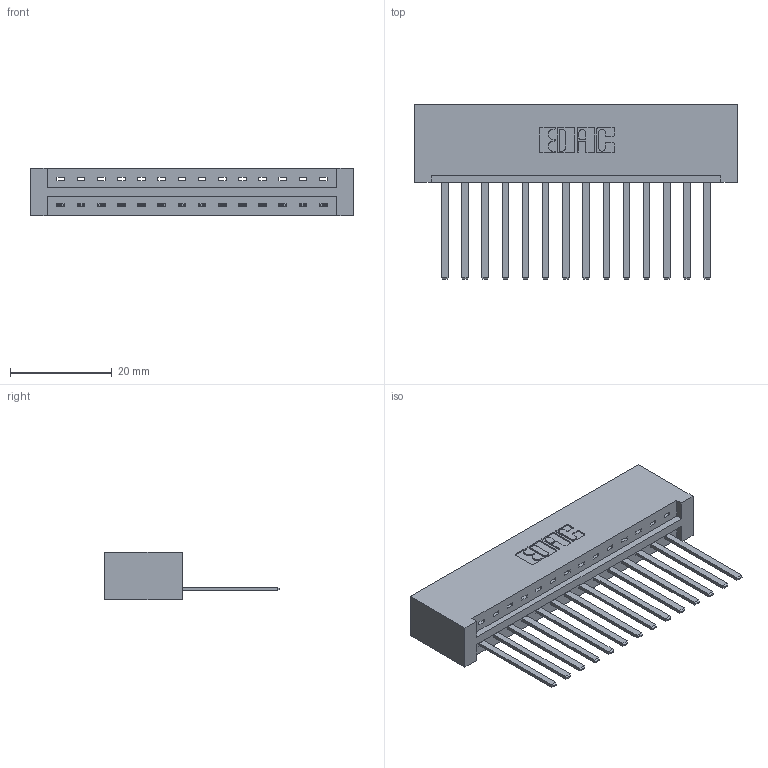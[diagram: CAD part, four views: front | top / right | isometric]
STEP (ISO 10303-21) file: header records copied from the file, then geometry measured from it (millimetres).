
FILE_DESCRIPTION (( 'STEP AP203' ), '1' );
FILE_NAME ('387-014-544-101.STEP', '2019-10-02T15:54:24', ( '' ), ( '' ), 'SwSTEP 2.0', 'SolidWorks 2016', '' );
FILE_SCHEMA (( 'CONFIG_CONTROL_DESIGN' ));
Length unit declared in the file: inch
Products named in the file (3): 337 Part_No Mounting Lugs; 345-292-001_345-293-144; 387-014-544-101
Assembly tree (15 placements, depth 2):
  387-014-544-101
    337 Part_No Mounting Lugs
    345-292-001_345-293-144  x14
Bounding box: 63.35 x 34.3 x 9.4 mm (x, y, z)
Volume: 7134.4 mm3; surface area: 7731.7 mm2
Topology: 15 solids, 15 shells, 890 faces, 2667 edges, 1758 vertices
Faces by surface type: plane 654, cylinder 236
Entity records: 13567 total; most frequent: CARTESIAN_POINT 2368, ORIENTED_EDGE 2318, DIRECTION 2039, EDGE_CURVE 1159, VECTOR 1043, LINE 1043, VERTEX_POINT 770, AXIS2_PLACEMENT_3D 498
